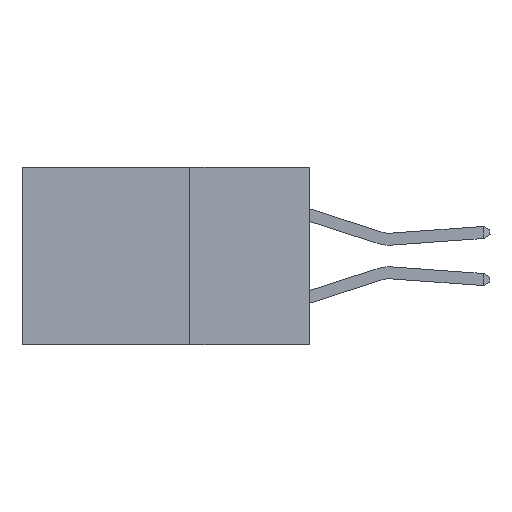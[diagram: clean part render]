
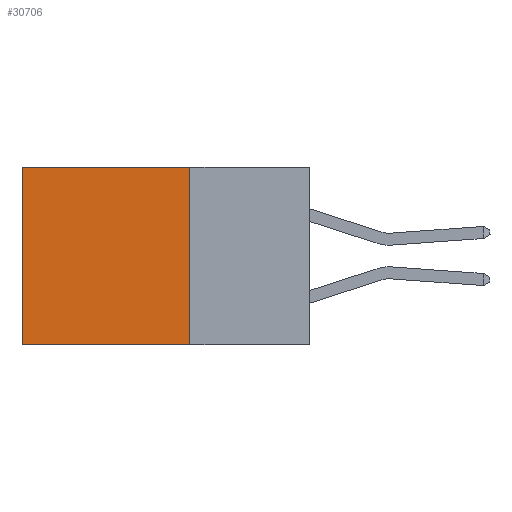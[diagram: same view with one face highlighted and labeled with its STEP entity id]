
A CAD part, left-side view. The second image highlights one B-rep face of the part: STEP entity #30706.
In plain terms, the highlighted planar face has unit normal (-1, 0, 0).
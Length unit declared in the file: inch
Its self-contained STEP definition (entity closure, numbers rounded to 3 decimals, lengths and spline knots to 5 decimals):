
#545 = DIRECTION ( 'NONE',  ( 0., 0., -1. ) ) ;
#1041 = LINE ( 'NONE', #3472, #21412 ) ;
#1409 = ORIENTED_EDGE ( 'NONE', *, *, #8076, .T. ) ;
#2027 = EDGE_CURVE ( 'NONE', #13305, #30567, #3516, .T. ) ;
#2909 = DIRECTION ( 'NONE',  ( 0., 1., 0. ) ) ;
#3472 = CARTESIAN_POINT ( 'NONE',  ( 0.298, 0.25, 0. ) ) ;
#3516 = LINE ( 'NONE', #5679, #16403 ) ;
#4494 = VERTEX_POINT ( 'NONE', #6849 ) ;
#5232 = VERTEX_POINT ( 'NONE', #23974 ) ;
#5679 = CARTESIAN_POINT ( 'NONE',  ( 0.298, 0.25, 0. ) ) ;
#6666 = ORIENTED_EDGE ( 'NONE', *, *, #8507, .F. ) ;
#6849 = CARTESIAN_POINT ( 'NONE',  ( 0.298, 0.6, -0.37 ) ) ;
#7662 = LINE ( 'NONE', #24051, #13053 ) ;
#8076 = EDGE_CURVE ( 'NONE', #30567, #4494, #7662, .T. ) ;
#8507 = EDGE_CURVE ( 'NONE', #5232, #4494, #33903, .T. ) ;
#11122 = DIRECTION ( 'NONE',  ( 0., 1., 0. ) ) ;
#11699 = ORIENTED_EDGE ( 'NONE', *, *, #2027, .T. ) ;
#13053 = VECTOR ( 'NONE', #27100, 39.37008 ) ;
#13305 = VERTEX_POINT ( 'NONE', #24419 ) ;
#13469 = CARTESIAN_POINT ( 'NONE',  ( 0.298, 0.25, -0.37 ) ) ;
#14593 = PLANE ( 'NONE',  #20092 ) ;
#16403 = VECTOR ( 'NONE', #11122, 39.37008 ) ;
#17270 = CARTESIAN_POINT ( 'NONE',  ( 0.298, 0.25, 0. ) ) ;
#18175 = FACE_OUTER_BOUND ( 'NONE', #24625, .T. ) ;
#19627 = EDGE_CURVE ( 'NONE', #13305, #5232, #1041, .T. ) ;
#20092 = AXIS2_PLACEMENT_3D ( 'NONE', #17270, #25306, #27973 ) ;
#21412 = VECTOR ( 'NONE', #545, 39.37008 ) ;
#23974 = CARTESIAN_POINT ( 'NONE',  ( 0.298, 0.25, -0.37 ) ) ;
#24051 = CARTESIAN_POINT ( 'NONE',  ( 0.298, 0.6, 0. ) ) ;
#24419 = CARTESIAN_POINT ( 'NONE',  ( 0.298, 0.25, 0. ) ) ;
#24625 = EDGE_LOOP ( 'NONE', ( #1409, #6666, #28268, #11699 ) ) ;
#25306 = DIRECTION ( 'NONE',  ( 1., 0., 0. ) ) ;
#27100 = DIRECTION ( 'NONE',  ( 0., 0., -1. ) ) ;
#27973 = DIRECTION ( 'NONE',  ( 0., 0., -1. ) ) ;
#28268 = ORIENTED_EDGE ( 'NONE', *, *, #19627, .F. ) ;
#30567 = VERTEX_POINT ( 'NONE', #33022 ) ;
#30706 = ADVANCED_FACE ( 'NONE', ( #18175 ), #14593, .F. ) ;
#30975 = VECTOR ( 'NONE', #2909, 39.37008 ) ;
#33022 = CARTESIAN_POINT ( 'NONE',  ( 0.298, 0.6, 0. ) ) ;
#33903 = LINE ( 'NONE', #13469, #30975 ) ;
